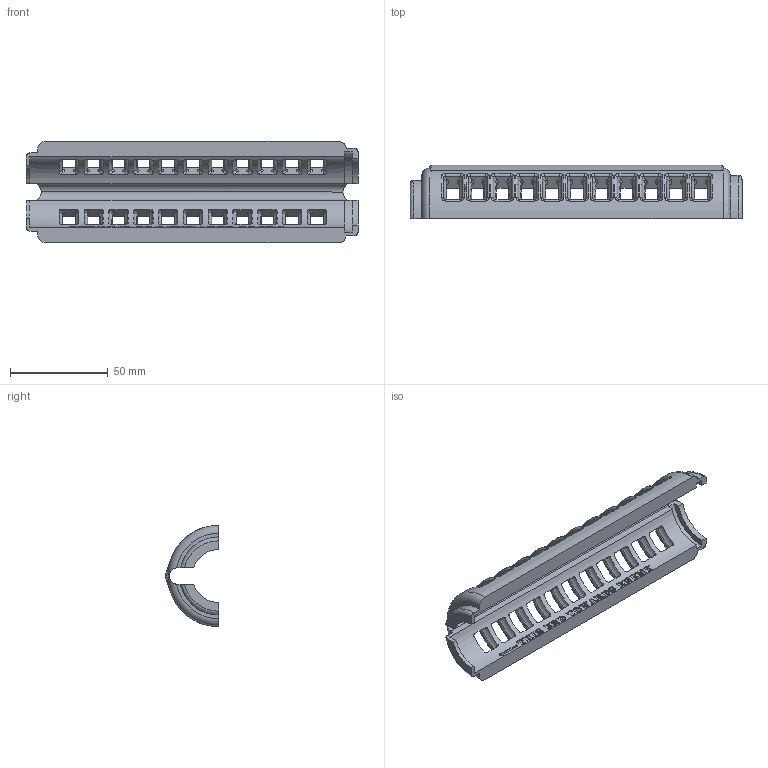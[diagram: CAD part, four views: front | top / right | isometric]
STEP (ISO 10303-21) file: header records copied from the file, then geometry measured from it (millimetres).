
FILE_DESCRIPTION (( 'STEP AP214' ), '1' );
FILE_NAME ('Carbine Handguard.STEP', '2014-02-06T10:17:13', ( 'elpi' ), ( '' ), 'SwSTEP 2.0', 'SolidWorks 2013', '' );
FILE_SCHEMA (( 'AUTOMOTIVE_DESIGN' ));
Length unit declared in the file: millimetre
Products named in the file (1): Carbine Handguard
Bounding box: 170 x 27.27 x 51.84 mm (x, y, z)
Volume: 59060.2 mm3; surface area: 30758.5 mm2
Topology: 1 solids, 1 shells, 1407 faces, 3695 edges, 2340 vertices
Faces by surface type: bspline 784, plane 281, torus 205, cylinder 137
Entity records: 69601 total; most frequent: CARTESIAN_POINT 40506, ORIENTED_EDGE 7386, DIRECTION 4091, EDGE_CURVE 3693, VERTEX_POINT 2340, B_SPLINE_CURVE_WITH_KNOTS 1660, AXIS2_PLACEMENT_3D 1560, EDGE_LOOP 1503
